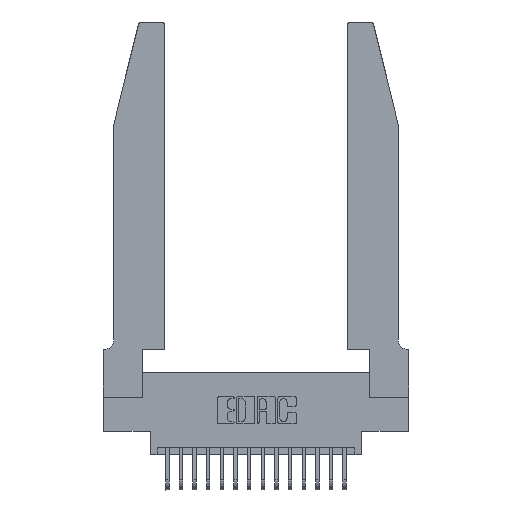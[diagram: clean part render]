
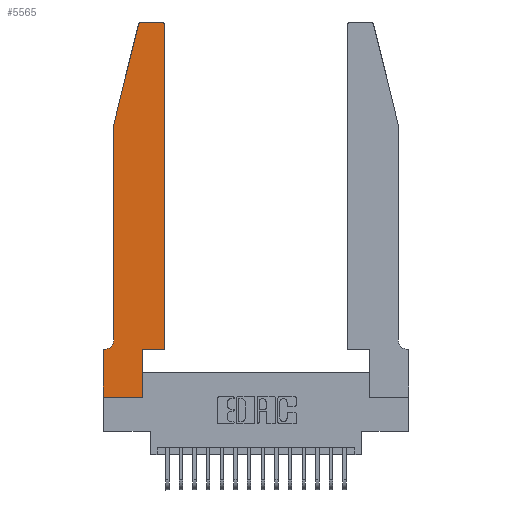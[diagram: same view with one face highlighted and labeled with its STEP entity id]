
A CAD part, top view. The second image highlights one B-rep face of the part: STEP entity #5565.
In plain terms, the highlighted planar face has unit normal (0, 0, 1).
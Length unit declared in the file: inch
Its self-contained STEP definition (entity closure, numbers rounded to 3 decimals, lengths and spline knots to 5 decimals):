
#264 = VERTEX_POINT ( 'NONE', #14527 ) ;
#453 = VERTEX_POINT ( 'NONE', #17471 ) ;
#674 = DIRECTION ( 'NONE',  ( -1., 0., 0. ) ) ;
#777 = DIRECTION ( 'NONE',  ( 0., 1., 0. ) ) ;
#883 = CARTESIAN_POINT ( 'NONE',  ( 0.4205, 2.75, 0.37 ) ) ;
#948 = DIRECTION ( 'NONE',  ( 0., 0., 1. ) ) ;
#1312 = ORIENTED_EDGE ( 'NONE', *, *, #2189, .T. ) ;
#1324 = DIRECTION ( 'NONE',  ( 1., 0., 0. ) ) ;
#1350 = FACE_OUTER_BOUND ( 'NONE', #13515, .T. ) ;
#1455 = LINE ( 'NONE', #3847, #8067 ) ;
#1694 = ORIENTED_EDGE ( 'NONE', *, *, #6712, .T. ) ;
#1822 = LINE ( 'NONE', #7919, #17181 ) ;
#2189 = EDGE_CURVE ( 'NONE', #7785, #11975, #1822, .T. ) ;
#2635 = EDGE_CURVE ( 'NONE', #9000, #14749, #19205, .T. ) ;
#2939 = ORIENTED_EDGE ( 'NONE', *, *, #5438, .T. ) ;
#3430 = ORIENTED_EDGE ( 'NONE', *, *, #17076, .T. ) ;
#3483 = EDGE_CURVE ( 'NONE', #11999, #9426, #13203, .T. ) ;
#3523 = DIRECTION ( 'NONE',  ( -0.239, -0.971, 0. ) ) ;
#3847 = CARTESIAN_POINT ( 'NONE',  ( 0.4505, 0.35, 0.37 ) ) ;
#4038 = EDGE_CURVE ( 'NONE', #5741, #453, #5332, .T. ) ;
#4051 = VERTEX_POINT ( 'NONE', #12414 ) ;
#5163 = VERTEX_POINT ( 'NONE', #5498 ) ;
#5332 = LINE ( 'NONE', #13921, #11341 ) ;
#5438 = EDGE_CURVE ( 'NONE', #4051, #7785, #9798, .T. ) ;
#5498 = CARTESIAN_POINT ( 'NONE',  ( 0., 0., 0.37 ) ) ;
#5565 = ADVANCED_FACE ( 'NONE', ( #1350 ), #17282, .T. ) ;
#5741 = VERTEX_POINT ( 'NONE', #19059 ) ;
#5897 = VECTOR ( 'NONE', #9484, 39.37008 ) ;
#6431 = DIRECTION ( 'NONE',  ( 1., 0., 0. ) ) ;
#6498 = CARTESIAN_POINT ( 'NONE',  ( 0., 0., 0.37 ) ) ;
#6712 = EDGE_CURVE ( 'NONE', #5163, #4051, #9062, .T. ) ;
#6813 = CARTESIAN_POINT ( 'NONE',  ( 0.0755, 2., 0.37 ) ) ;
#6826 = EDGE_CURVE ( 'NONE', #9426, #5741, #11150, .T. ) ;
#7148 = VECTOR ( 'NONE', #16092, 39.37008 ) ;
#7188 = CARTESIAN_POINT ( 'NONE',  ( 0.0055, 0.35, 0.37 ) ) ;
#7481 = CARTESIAN_POINT ( 'NONE',  ( 0.2865, 0.35, 0.37 ) ) ;
#7653 = CIRCLE ( 'NONE', #13666, 0.03 ) ;
#7785 = VERTEX_POINT ( 'NONE', #7481 ) ;
#7841 = CARTESIAN_POINT ( 'NONE',  ( 0.0055, 0.42, 0.37 ) ) ;
#7919 = CARTESIAN_POINT ( 'NONE',  ( 0.4505, 0.35, 0.37 ) ) ;
#8029 = ORIENTED_EDGE ( 'NONE', *, *, #4038, .T. ) ;
#8067 = VECTOR ( 'NONE', #777, 39.37008 ) ;
#8284 = DIRECTION ( 'NONE',  ( 0., 0., 1. ) ) ;
#8459 = CARTESIAN_POINT ( 'NONE',  ( 0., 0.35, 0.37 ) ) ;
#8607 = VECTOR ( 'NONE', #13919, 39.37008 ) ;
#8947 = LINE ( 'NONE', #12585, #9401 ) ;
#9000 = VERTEX_POINT ( 'NONE', #16567 ) ;
#9062 = LINE ( 'NONE', #6498, #8607 ) ;
#9309 = DIRECTION ( 'NONE',  ( -1., 0., 0. ) ) ;
#9401 = VECTOR ( 'NONE', #674, 39.37008 ) ;
#9426 = VERTEX_POINT ( 'NONE', #14547 ) ;
#9484 = DIRECTION ( 'NONE',  ( 0., 1., 0. ) ) ;
#9597 = ORIENTED_EDGE ( 'NONE', *, *, #2635, .T. ) ;
#9798 = LINE ( 'NONE', #13897, #5897 ) ;
#10311 = DIRECTION ( 'NONE',  ( 0., 0., 1. ) ) ;
#11150 = CIRCLE ( 'NONE', #12810, 0.03 ) ;
#11341 = VECTOR ( 'NONE', #3523, 39.37008 ) ;
#11428 = DIRECTION ( 'NONE',  ( 1., 0., 0. ) ) ;
#11659 = ORIENTED_EDGE ( 'NONE', *, *, #6826, .T. ) ;
#11911 = ORIENTED_EDGE ( 'NONE', *, *, #17622, .T. ) ;
#11975 = VERTEX_POINT ( 'NONE', #17155 ) ;
#11999 = VERTEX_POINT ( 'NONE', #883 ) ;
#12414 = CARTESIAN_POINT ( 'NONE',  ( 0.2865, 0., 0.37 ) ) ;
#12585 = CARTESIAN_POINT ( 'NONE',  ( 0.0755, 0.35, 0.37 ) ) ;
#12646 = AXIS2_PLACEMENT_3D ( 'NONE', #7841, #18119, #9309 ) ;
#12696 = CARTESIAN_POINT ( 'NONE',  ( 0.2605, 2.75, 0.37 ) ) ;
#12745 = VECTOR ( 'NONE', #15681, 39.37008 ) ;
#12810 = AXIS2_PLACEMENT_3D ( 'NONE', #17123, #8284, #18580 ) ;
#13203 = LINE ( 'NONE', #12696, #12745 ) ;
#13515 = EDGE_LOOP ( 'NONE', ( #17298, #11659, #8029, #18064, #9597, #14510, #11911, #1694, #2939, #1312, #3430, #18539 ) ) ;
#13666 = AXIS2_PLACEMENT_3D ( 'NONE', #19104, #10311, #1324 ) ;
#13718 = VERTEX_POINT ( 'NONE', #16620 ) ;
#13897 = CARTESIAN_POINT ( 'NONE',  ( 0.2865, 0.35, 0.37 ) ) ;
#13919 = DIRECTION ( 'NONE',  ( 1., 0., 0. ) ) ;
#13921 = CARTESIAN_POINT ( 'NONE',  ( 0.0755, 2., 0.37 ) ) ;
#14510 = ORIENTED_EDGE ( 'NONE', *, *, #17954, .T. ) ;
#14527 = CARTESIAN_POINT ( 'NONE',  ( 0., 0.35, 0.37 ) ) ;
#14547 = CARTESIAN_POINT ( 'NONE',  ( 0.284, 2.75, 0.37 ) ) ;
#14749 = VERTEX_POINT ( 'NONE', #7188 ) ;
#15681 = DIRECTION ( 'NONE',  ( -1., 0., 0. ) ) ;
#16092 = DIRECTION ( 'NONE',  ( 0., -1., 0. ) ) ;
#16567 = CARTESIAN_POINT ( 'NONE',  ( 0.0755, 0.42, 0.37 ) ) ;
#16620 = CARTESIAN_POINT ( 'NONE',  ( 0.4505, 2.72, 0.37 ) ) ;
#16686 = EDGE_CURVE ( 'NONE', #13718, #11999, #7653, .T. ) ;
#17076 = EDGE_CURVE ( 'NONE', #11975, #13718, #1455, .T. ) ;
#17115 = DIRECTION ( 'NONE',  ( 0., -1., 0. ) ) ;
#17123 = CARTESIAN_POINT ( 'NONE',  ( 0.284, 2.72, 0.37 ) ) ;
#17155 = CARTESIAN_POINT ( 'NONE',  ( 0.4505, 0.35, 0.37 ) ) ;
#17181 = VECTOR ( 'NONE', #6431, 39.37008 ) ;
#17282 = PLANE ( 'NONE',  #19196 ) ;
#17298 = ORIENTED_EDGE ( 'NONE', *, *, #3483, .T. ) ;
#17434 = EDGE_CURVE ( 'NONE', #453, #9000, #18174, .T. ) ;
#17471 = CARTESIAN_POINT ( 'NONE',  ( 0.0755, 2., 0.37 ) ) ;
#17539 = CARTESIAN_POINT ( 'NONE',  ( 0., 0., 0.37 ) ) ;
#17622 = EDGE_CURVE ( 'NONE', #264, #5163, #18856, .T. ) ;
#17727 = VECTOR ( 'NONE', #17115, 39.37008 ) ;
#17954 = EDGE_CURVE ( 'NONE', #14749, #264, #8947, .T. ) ;
#18064 = ORIENTED_EDGE ( 'NONE', *, *, #17434, .T. ) ;
#18119 = DIRECTION ( 'NONE',  ( 0., 0., -1. ) ) ;
#18174 = LINE ( 'NONE', #6813, #17727 ) ;
#18539 = ORIENTED_EDGE ( 'NONE', *, *, #16686, .T. ) ;
#18580 = DIRECTION ( 'NONE',  ( 1., 0., 0. ) ) ;
#18856 = LINE ( 'NONE', #17539, #7148 ) ;
#19059 = CARTESIAN_POINT ( 'NONE',  ( 0.25487, 2.72718, 0.37 ) ) ;
#19104 = CARTESIAN_POINT ( 'NONE',  ( 0.4205, 2.72, 0.37 ) ) ;
#19196 = AXIS2_PLACEMENT_3D ( 'NONE', #8459, #948, #11428 ) ;
#19205 = CIRCLE ( 'NONE', #12646, 0.07 ) ;
